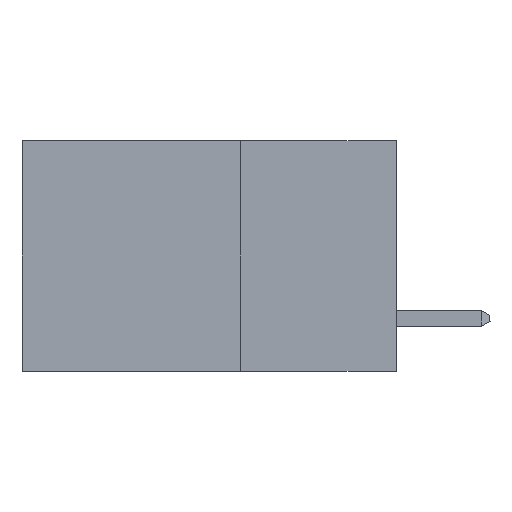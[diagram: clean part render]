
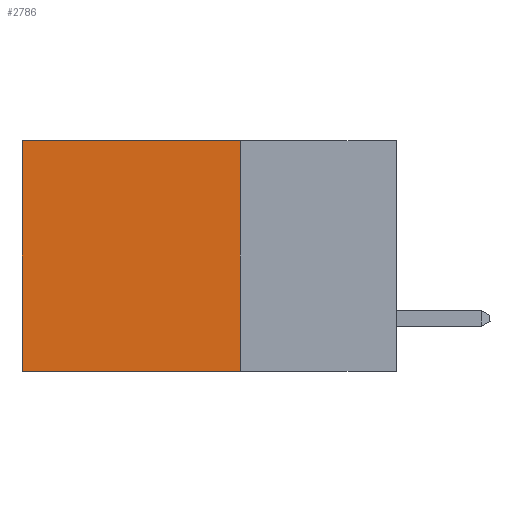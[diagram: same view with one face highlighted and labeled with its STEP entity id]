
A CAD part, left-side view. The second image highlights one B-rep face of the part: STEP entity #2786.
In plain terms, the highlighted planar face has unit normal (-1, 0, 0).
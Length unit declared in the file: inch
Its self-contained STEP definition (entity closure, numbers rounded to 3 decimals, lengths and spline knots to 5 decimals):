
#259 = ORIENTED_EDGE ( 'NONE', *, *, #2020, .T. ) ;
#350 = CARTESIAN_POINT ( 'NONE',  ( 0.298, 0.6, 0. ) ) ;
#619 = LINE ( 'NONE', #8478, #7584 ) ;
#723 = FACE_OUTER_BOUND ( 'NONE', #838, .T. ) ;
#838 = EDGE_LOOP ( 'NONE', ( #259, #1048, #4291, #6899 ) ) ;
#1048 = ORIENTED_EDGE ( 'NONE', *, *, #6648, .F. ) ;
#1807 = AXIS2_PLACEMENT_3D ( 'NONE', #3381, #4961, #4727 ) ;
#1924 = CARTESIAN_POINT ( 'NONE',  ( 0.298, 0.6, -0.37 ) ) ;
#2020 = EDGE_CURVE ( 'NONE', #8483, #9475, #619, .T. ) ;
#2336 = VERTEX_POINT ( 'NONE', #6716 ) ;
#2786 = ADVANCED_FACE ( 'NONE', ( #723 ), #3985, .F. ) ;
#2944 = CARTESIAN_POINT ( 'NONE',  ( 0.298, 0.25, 0. ) ) ;
#3265 = LINE ( 'NONE', #9464, #5041 ) ;
#3319 = CARTESIAN_POINT ( 'NONE',  ( 0.298, 0.25, -0.37 ) ) ;
#3381 = CARTESIAN_POINT ( 'NONE',  ( 0.298, 0.25, 0. ) ) ;
#3832 = EDGE_CURVE ( 'NONE', #4993, #2336, #3265, .T. ) ;
#3938 = VECTOR ( 'NONE', #4931, 39.37008 ) ;
#3985 = PLANE ( 'NONE',  #1807 ) ;
#4291 = ORIENTED_EDGE ( 'NONE', *, *, #3832, .F. ) ;
#4632 = LINE ( 'NONE', #3319, #3938 ) ;
#4727 = DIRECTION ( 'NONE',  ( 0., 0., -1. ) ) ;
#4741 = DIRECTION ( 'NONE',  ( 0., 0., -1. ) ) ;
#4931 = DIRECTION ( 'NONE',  ( 0., 1., 0. ) ) ;
#4932 = VECTOR ( 'NONE', #7329, 39.37008 ) ;
#4961 = DIRECTION ( 'NONE',  ( 1., 0., 0. ) ) ;
#4993 = VERTEX_POINT ( 'NONE', #5853 ) ;
#5041 = VECTOR ( 'NONE', #6599, 39.37008 ) ;
#5179 = LINE ( 'NONE', #2944, #4932 ) ;
#5853 = CARTESIAN_POINT ( 'NONE',  ( 0.298, 0.25, 0. ) ) ;
#6599 = DIRECTION ( 'NONE',  ( 0., 0., -1. ) ) ;
#6648 = EDGE_CURVE ( 'NONE', #2336, #9475, #4632, .T. ) ;
#6716 = CARTESIAN_POINT ( 'NONE',  ( 0.298, 0.25, -0.37 ) ) ;
#6899 = ORIENTED_EDGE ( 'NONE', *, *, #9185, .T. ) ;
#7329 = DIRECTION ( 'NONE',  ( 0., 1., 0. ) ) ;
#7584 = VECTOR ( 'NONE', #4741, 39.37008 ) ;
#8478 = CARTESIAN_POINT ( 'NONE',  ( 0.298, 0.6, 0. ) ) ;
#8483 = VERTEX_POINT ( 'NONE', #350 ) ;
#9185 = EDGE_CURVE ( 'NONE', #4993, #8483, #5179, .T. ) ;
#9464 = CARTESIAN_POINT ( 'NONE',  ( 0.298, 0.25, 0. ) ) ;
#9475 = VERTEX_POINT ( 'NONE', #1924 ) ;
